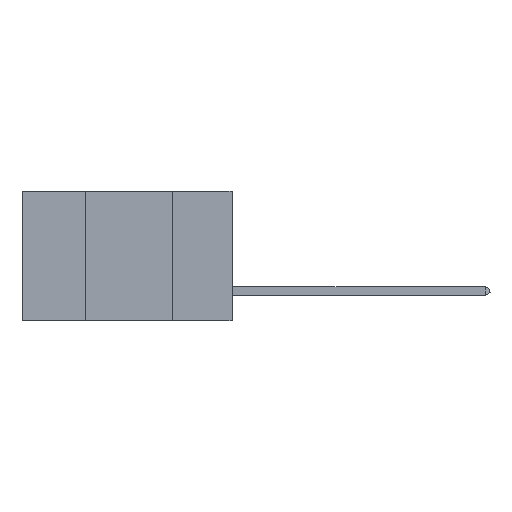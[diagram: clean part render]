
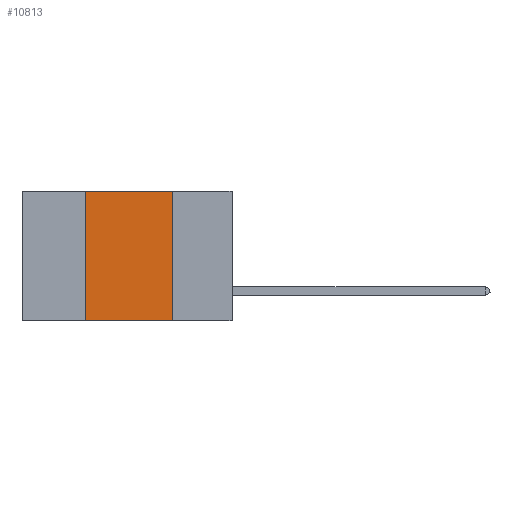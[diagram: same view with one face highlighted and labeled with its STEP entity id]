
A CAD part, left-side view. The second image highlights one B-rep face of the part: STEP entity #10813.
In plain terms, the highlighted planar face has unit normal (-1, 0, 0).
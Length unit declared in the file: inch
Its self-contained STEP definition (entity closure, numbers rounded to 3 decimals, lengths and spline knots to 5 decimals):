
#441 = ORIENTED_EDGE ( 'NONE', *, *, #17512, .F. ) ;
#935 = VECTOR ( 'NONE', #10519, 39.37008 ) ;
#1132 = VERTEX_POINT ( 'NONE', #11954 ) ;
#1498 = CARTESIAN_POINT ( 'NONE',  ( 0., 0.6, 0. ) ) ;
#1687 = CARTESIAN_POINT ( 'NONE',  ( 0., 0.42, 0. ) ) ;
#1820 = ORIENTED_EDGE ( 'NONE', *, *, #14169, .F. ) ;
#2433 = CARTESIAN_POINT ( 'NONE',  ( 0., 0.42, -0.37 ) ) ;
#2488 = ORIENTED_EDGE ( 'NONE', *, *, #18839, .F. ) ;
#4142 = DIRECTION ( 'NONE',  ( 0., 0., -1. ) ) ;
#6658 = EDGE_LOOP ( 'NONE', ( #441, #2488, #1820, #8909 ) ) ;
#8680 = AXIS2_PLACEMENT_3D ( 'NONE', #15976, #19293, #4142 ) ;
#8851 = VERTEX_POINT ( 'NONE', #1687 ) ;
#8909 = ORIENTED_EDGE ( 'NONE', *, *, #16558, .T. ) ;
#9447 = FACE_OUTER_BOUND ( 'NONE', #6658, .T. ) ;
#10375 = CARTESIAN_POINT ( 'NONE',  ( 0., 0.42, 0. ) ) ;
#10519 = DIRECTION ( 'NONE',  ( 0., 0., 1. ) ) ;
#10813 = ADVANCED_FACE ( 'NONE', ( #9447 ), #12591, .F. ) ;
#11019 = CARTESIAN_POINT ( 'NONE',  ( 0., 0.17, 0. ) ) ;
#11119 = VERTEX_POINT ( 'NONE', #2433 ) ;
#11351 = LINE ( 'NONE', #13293, #21544 ) ;
#11405 = DIRECTION ( 'NONE',  ( 0., 0., -1. ) ) ;
#11879 = VERTEX_POINT ( 'NONE', #11019 ) ;
#11954 = CARTESIAN_POINT ( 'NONE',  ( 0., 0.17, -0.37 ) ) ;
#12591 = PLANE ( 'NONE',  #8680 ) ;
#12596 = VECTOR ( 'NONE', #21275, 39.37008 ) ;
#13293 = CARTESIAN_POINT ( 'NONE',  ( 0., 0.17, 0. ) ) ;
#14169 = EDGE_CURVE ( 'NONE', #11119, #8851, #20748, .T. ) ;
#15976 = CARTESIAN_POINT ( 'NONE',  ( 0., 0.6, 0. ) ) ;
#16558 = EDGE_CURVE ( 'NONE', #11119, #1132, #17261, .T. ) ;
#16767 = VECTOR ( 'NONE', #20387, 39.37008 ) ;
#17261 = LINE ( 'NONE', #20595, #16767 ) ;
#17512 = EDGE_CURVE ( 'NONE', #11879, #1132, #11351, .T. ) ;
#18839 = EDGE_CURVE ( 'NONE', #8851, #11879, #18843, .T. ) ;
#18843 = LINE ( 'NONE', #1498, #12596 ) ;
#19293 = DIRECTION ( 'NONE',  ( 1., 0., 0. ) ) ;
#20387 = DIRECTION ( 'NONE',  ( 0., -1., 0. ) ) ;
#20595 = CARTESIAN_POINT ( 'NONE',  ( 0., 0.6, -0.37 ) ) ;
#20748 = LINE ( 'NONE', #10375, #935 ) ;
#21275 = DIRECTION ( 'NONE',  ( 0., -1., 0. ) ) ;
#21544 = VECTOR ( 'NONE', #11405, 39.37008 ) ;
